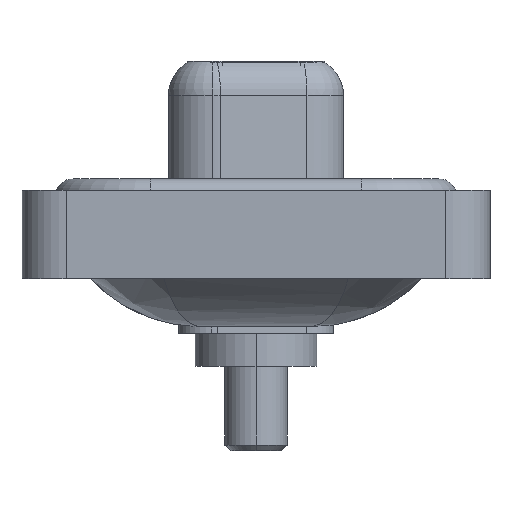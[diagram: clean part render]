
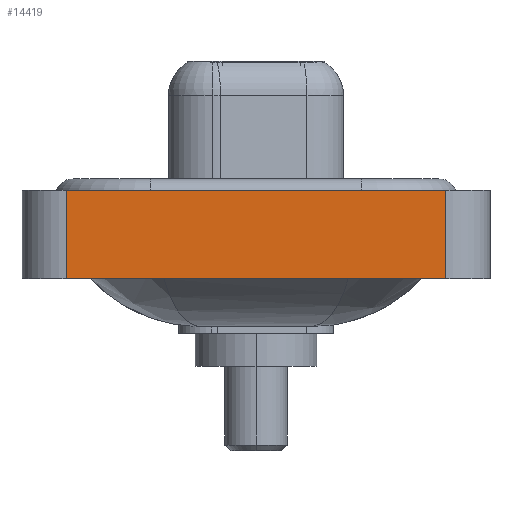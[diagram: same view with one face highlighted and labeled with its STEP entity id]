
A CAD part, left-side view. The second image highlights one B-rep face of the part: STEP entity #14419.
In plain terms, the highlighted planar face has unit normal (-1, 0, 0).
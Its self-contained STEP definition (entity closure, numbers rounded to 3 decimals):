
#152 = FACE_OUTER_BOUND ( 'NONE', #12183, .T. ) ;
#371 = EDGE_CURVE ( 'NONE', #10313, #2332, #12425, .T. ) ;
#543 = VECTOR ( 'NONE', #14890, 1000. ) ;
#1267 = DIRECTION ( 'NONE',  ( 0., -1., 0. ) ) ;
#1354 = CARTESIAN_POINT ( 'NONE',  ( -7.25, -8.55, -3.6 ) ) ;
#2332 = VERTEX_POINT ( 'NONE', #15221 ) ;
#2962 = ORIENTED_EDGE ( 'NONE', *, *, #12840, .F. ) ;
#3317 = VECTOR ( 'NONE', #11971, 1000. ) ;
#3386 = VERTEX_POINT ( 'NONE', #10266 ) ;
#4467 = ORIENTED_EDGE ( 'NONE', *, *, #15863, .T. ) ;
#4837 = CARTESIAN_POINT ( 'NONE',  ( -7.25, 8.55, -3.6 ) ) ;
#5120 = ORIENTED_EDGE ( 'NONE', *, *, #371, .F. ) ;
#6162 = CARTESIAN_POINT ( 'NONE',  ( -7.25, 8.55, -3.6 ) ) ;
#6450 = EDGE_CURVE ( 'NONE', #3386, #7611, #12872, .T. ) ;
#7008 = CARTESIAN_POINT ( 'NONE',  ( -7.25, -8.55, -3.6 ) ) ;
#7287 = VECTOR ( 'NONE', #1267, 1000. ) ;
#7606 = PLANE ( 'NONE',  #10572 ) ;
#7611 = VERTEX_POINT ( 'NONE', #7914 ) ;
#7914 = CARTESIAN_POINT ( 'NONE',  ( -7.25, -8.55, 0.4 ) ) ;
#7961 = ORIENTED_EDGE ( 'NONE', *, *, #6450, .T. ) ;
#8633 = CARTESIAN_POINT ( 'NONE',  ( -7.25, -8.55, 0.4 ) ) ;
#10181 = CARTESIAN_POINT ( 'NONE',  ( -7.25, -8.55, -3.6 ) ) ;
#10258 = LINE ( 'NONE', #10181, #543 ) ;
#10266 = CARTESIAN_POINT ( 'NONE',  ( -7.25, -8.55, -3.6 ) ) ;
#10313 = VERTEX_POINT ( 'NONE', #4837 ) ;
#10572 = AXIS2_PLACEMENT_3D ( 'NONE', #1354, #14810, #11287 ) ;
#11275 = LINE ( 'NONE', #8633, #7287 ) ;
#11287 = DIRECTION ( 'NONE',  ( 0., 0., 1. ) ) ;
#11971 = DIRECTION ( 'NONE',  ( 0., 0., 1. ) ) ;
#12183 = EDGE_LOOP ( 'NONE', ( #7961, #2962, #5120, #4467 ) ) ;
#12425 = LINE ( 'NONE', #6162, #12593 ) ;
#12593 = VECTOR ( 'NONE', #14749, 1000. ) ;
#12840 = EDGE_CURVE ( 'NONE', #2332, #7611, #11275, .T. ) ;
#12872 = LINE ( 'NONE', #7008, #3317 ) ;
#14419 = ADVANCED_FACE ( 'NONE', ( #152 ), #7606, .T. ) ;
#14749 = DIRECTION ( 'NONE',  ( 0., 0., 1. ) ) ;
#14810 = DIRECTION ( 'NONE',  ( -1., 0., 0. ) ) ;
#14890 = DIRECTION ( 'NONE',  ( 0., -1., 0. ) ) ;
#15221 = CARTESIAN_POINT ( 'NONE',  ( -7.25, 8.55, 0.4 ) ) ;
#15863 = EDGE_CURVE ( 'NONE', #10313, #3386, #10258, .T. ) ;
